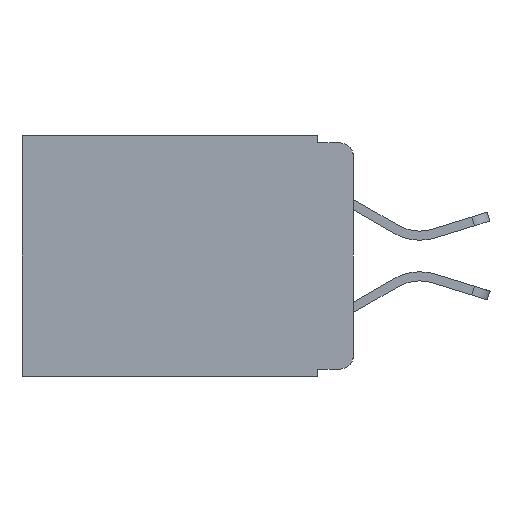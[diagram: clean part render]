
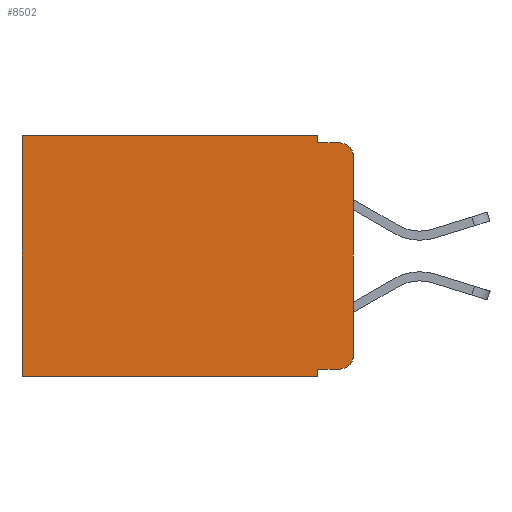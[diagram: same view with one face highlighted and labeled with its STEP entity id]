
A CAD part, left-side view. The second image highlights one B-rep face of the part: STEP entity #8502.
In plain terms, the highlighted planar face has unit normal (-1, 0, 0).
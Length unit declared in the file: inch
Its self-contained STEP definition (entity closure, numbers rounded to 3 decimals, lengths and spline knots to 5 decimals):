
#2 = EDGE_CURVE ( 'NONE', #5339, #12790, #4103, .T. ) ;
#128 = ORIENTED_EDGE ( 'NONE', *, *, #14231, .F. ) ;
#335 = CARTESIAN_POINT ( 'NONE',  ( 0.298, 0.051, 0. ) ) ;
#374 = PLANE ( 'NONE',  #11305 ) ;
#831 = CARTESIAN_POINT ( 'NONE',  ( 0.298, 0., -0.313 ) ) ;
#932 = VECTOR ( 'NONE', #6007, 39.37008 ) ;
#953 = CARTESIAN_POINT ( 'NONE',  ( 0.298, 0.051, 0. ) ) ;
#1104 = EDGE_CURVE ( 'NONE', #4106, #7980, #6738, .T. ) ;
#1305 = CARTESIAN_POINT ( 'NONE',  ( 0.298, 0.02, -0.333 ) ) ;
#1593 = CARTESIAN_POINT ( 'NONE',  ( 0.298, 0.02, -0.01 ) ) ;
#1786 = EDGE_CURVE ( 'NONE', #9860, #7980, #3291, .T. ) ;
#1816 = EDGE_CURVE ( 'NONE', #13591, #5136, #9342, .T. ) ;
#1869 = CARTESIAN_POINT ( 'NONE',  ( 0.298, 0., -0.343 ) ) ;
#1994 = DIRECTION ( 'NONE',  ( 0., -1., 0. ) ) ;
#2208 = CARTESIAN_POINT ( 'NONE',  ( 0.298, 0.02, -0.03 ) ) ;
#2217 = CARTESIAN_POINT ( 'NONE',  ( 0.298, 0.473, 0. ) ) ;
#2262 = DIRECTION ( 'NONE',  ( 0., 0., -1. ) ) ;
#2294 = LINE ( 'NONE', #4099, #15193 ) ;
#2522 = ORIENTED_EDGE ( 'NONE', *, *, #7919, .T. ) ;
#2670 = ORIENTED_EDGE ( 'NONE', *, *, #10797, .T. ) ;
#2730 = CIRCLE ( 'NONE', #14748, 0.02 ) ;
#2854 = CARTESIAN_POINT ( 'NONE',  ( 0.298, 0., 0. ) ) ;
#2882 = ORIENTED_EDGE ( 'NONE', *, *, #1786, .T. ) ;
#3291 = LINE ( 'NONE', #6824, #8205 ) ;
#3305 = ORIENTED_EDGE ( 'NONE', *, *, #5831, .F. ) ;
#3557 = CARTESIAN_POINT ( 'NONE',  ( 0.298, 0.051, -0.01 ) ) ;
#3772 = CIRCLE ( 'NONE', #7997, 0.02 ) ;
#4076 = DIRECTION ( 'NONE',  ( 0., 0., -1. ) ) ;
#4099 = CARTESIAN_POINT ( 'NONE',  ( 0.298, 0.051, 0. ) ) ;
#4103 = LINE ( 'NONE', #3557, #932 ) ;
#4106 = VERTEX_POINT ( 'NONE', #5412 ) ;
#4938 = ORIENTED_EDGE ( 'NONE', *, *, #7126, .T. ) ;
#5136 = VERTEX_POINT ( 'NONE', #1305 ) ;
#5339 = VERTEX_POINT ( 'NONE', #8785 ) ;
#5412 = CARTESIAN_POINT ( 'NONE',  ( 0.298, 0.051, -0.343 ) ) ;
#5595 = DIRECTION ( 'NONE',  ( -1., 0., 0. ) ) ;
#5762 = DIRECTION ( 'NONE',  ( 0., 0., -1. ) ) ;
#5831 = EDGE_CURVE ( 'NONE', #13591, #4106, #15143, .T. ) ;
#5888 = VECTOR ( 'NONE', #8601, 39.37008 ) ;
#6007 = DIRECTION ( 'NONE',  ( 0., -1., 0. ) ) ;
#6355 = CARTESIAN_POINT ( 'NONE',  ( 0.298, 0., 0. ) ) ;
#6655 = EDGE_LOOP ( 'NONE', ( #128, #4938, #12861, #13775, #2522, #2882, #9181, #3305, #10496, #2670 ) ) ;
#6702 = VERTEX_POINT ( 'NONE', #335 ) ;
#6738 = LINE ( 'NONE', #1869, #11657 ) ;
#6824 = CARTESIAN_POINT ( 'NONE',  ( 0.298, 0.473, 0. ) ) ;
#7126 = EDGE_CURVE ( 'NONE', #9164, #12790, #2730, .T. ) ;
#7520 = VECTOR ( 'NONE', #9386, 39.37008 ) ;
#7713 = CARTESIAN_POINT ( 'NONE',  ( 0.298, 0.473, -0.343 ) ) ;
#7919 = EDGE_CURVE ( 'NONE', #6702, #9860, #11649, .T. ) ;
#7980 = VERTEX_POINT ( 'NONE', #7713 ) ;
#7997 = AXIS2_PLACEMENT_3D ( 'NONE', #13025, #5595, #5762 ) ;
#8205 = VECTOR ( 'NONE', #14096, 39.37008 ) ;
#8502 = ADVANCED_FACE ( 'NONE', ( #11423 ), #374, .F. ) ;
#8601 = DIRECTION ( 'NONE',  ( 0., 0., -1. ) ) ;
#8605 = VERTEX_POINT ( 'NONE', #831 ) ;
#8785 = CARTESIAN_POINT ( 'NONE',  ( 0.298, 0.051, -0.01 ) ) ;
#8863 = DIRECTION ( 'NONE',  ( 0., 1., 0. ) ) ;
#9164 = VERTEX_POINT ( 'NONE', #12597 ) ;
#9181 = ORIENTED_EDGE ( 'NONE', *, *, #1104, .F. ) ;
#9279 = LINE ( 'NONE', #15547, #5888 ) ;
#9342 = LINE ( 'NONE', #13979, #12567 ) ;
#9347 = VECTOR ( 'NONE', #8863, 39.37008 ) ;
#9386 = DIRECTION ( 'NONE',  ( 0., 0., -1. ) ) ;
#9602 = DIRECTION ( 'NONE',  ( -1., 0., 0. ) ) ;
#9860 = VERTEX_POINT ( 'NONE', #2217 ) ;
#10326 = DIRECTION ( 'NONE',  ( 0., 1., 0. ) ) ;
#10496 = ORIENTED_EDGE ( 'NONE', *, *, #1816, .T. ) ;
#10628 = EDGE_CURVE ( 'NONE', #6702, #5339, #2294, .T. ) ;
#10797 = EDGE_CURVE ( 'NONE', #5136, #8605, #3772, .T. ) ;
#11253 = DIRECTION ( 'NONE',  ( 1., 0., 0. ) ) ;
#11305 = AXIS2_PLACEMENT_3D ( 'NONE', #2854, #11253, #4076 ) ;
#11423 = FACE_OUTER_BOUND ( 'NONE', #6655, .T. ) ;
#11649 = LINE ( 'NONE', #6355, #9347 ) ;
#11657 = VECTOR ( 'NONE', #10326, 39.37008 ) ;
#12567 = VECTOR ( 'NONE', #1994, 39.37008 ) ;
#12597 = CARTESIAN_POINT ( 'NONE',  ( 0.298, 0., -0.03 ) ) ;
#12790 = VERTEX_POINT ( 'NONE', #1593 ) ;
#12861 = ORIENTED_EDGE ( 'NONE', *, *, #2, .F. ) ;
#13025 = CARTESIAN_POINT ( 'NONE',  ( 0.298, 0.02, -0.313 ) ) ;
#13591 = VERTEX_POINT ( 'NONE', #14632 ) ;
#13775 = ORIENTED_EDGE ( 'NONE', *, *, #10628, .F. ) ;
#13979 = CARTESIAN_POINT ( 'NONE',  ( 0.298, 0.051, -0.333 ) ) ;
#14096 = DIRECTION ( 'NONE',  ( 0., 0., -1. ) ) ;
#14231 = EDGE_CURVE ( 'NONE', #9164, #8605, #9279, .T. ) ;
#14632 = CARTESIAN_POINT ( 'NONE',  ( 0.298, 0.051, -0.333 ) ) ;
#14748 = AXIS2_PLACEMENT_3D ( 'NONE', #2208, #9602, #2262 ) ;
#15104 = DIRECTION ( 'NONE',  ( 0., 0., -1. ) ) ;
#15143 = LINE ( 'NONE', #953, #7520 ) ;
#15193 = VECTOR ( 'NONE', #15104, 39.37008 ) ;
#15547 = CARTESIAN_POINT ( 'NONE',  ( 0.298, 0., 0. ) ) ;
